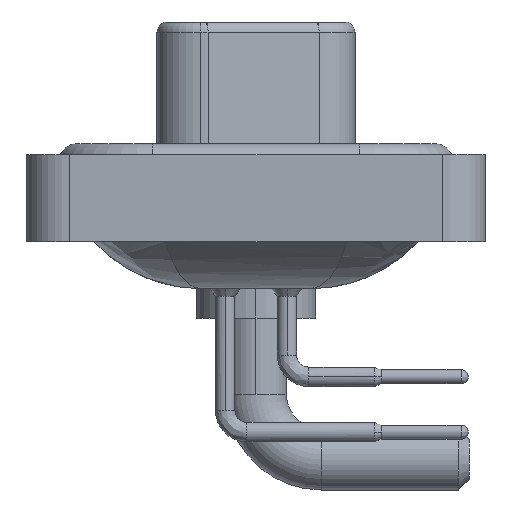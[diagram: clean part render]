
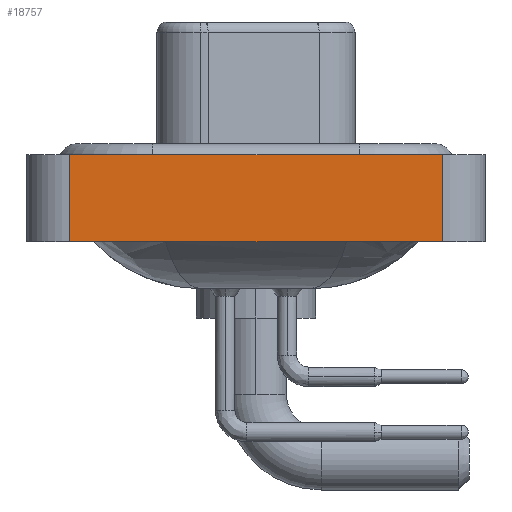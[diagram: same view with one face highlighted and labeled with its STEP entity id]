
A CAD part, left-side view. The second image highlights one B-rep face of the part: STEP entity #18757.
In plain terms, the highlighted planar face has unit normal (-1, 0, 0).
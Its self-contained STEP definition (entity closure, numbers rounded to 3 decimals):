
#782 = CARTESIAN_POINT ( 'NONE',  ( -7.35, -8.55, -3.6 ) ) ;
#877 = CARTESIAN_POINT ( 'NONE',  ( -7.35, -8.55, -3.6 ) ) ;
#1159 = CARTESIAN_POINT ( 'NONE',  ( -7.35, 8.55, 0.4 ) ) ;
#2008 = DIRECTION ( 'NONE',  ( 0., 0., 1. ) ) ;
#2098 = ORIENTED_EDGE ( 'NONE', *, *, #25594, .F. ) ;
#3463 = VERTEX_POINT ( 'NONE', #29595 ) ;
#3980 = LINE ( 'NONE', #877, #20474 ) ;
#4393 = LINE ( 'NONE', #14149, #15661 ) ;
#4493 = CARTESIAN_POINT ( 'NONE',  ( -7.35, -8.55, -3.6 ) ) ;
#5490 = VERTEX_POINT ( 'NONE', #4493 ) ;
#5574 = DIRECTION ( 'NONE',  ( -1., 0., 0. ) ) ;
#5680 = ORIENTED_EDGE ( 'NONE', *, *, #21581, .T. ) ;
#6449 = VERTEX_POINT ( 'NONE', #9210 ) ;
#6730 = EDGE_CURVE ( 'NONE', #5490, #6449, #8735, .T. ) ;
#7424 = VERTEX_POINT ( 'NONE', #1159 ) ;
#8735 = LINE ( 'NONE', #26713, #27895 ) ;
#9210 = CARTESIAN_POINT ( 'NONE',  ( -7.35, -8.55, 0.4 ) ) ;
#9489 = DIRECTION ( 'NONE',  ( 0., 0., 1. ) ) ;
#11653 = EDGE_LOOP ( 'NONE', ( #24681, #23798, #2098, #5680 ) ) ;
#13937 = AXIS2_PLACEMENT_3D ( 'NONE', #782, #5574, #9489 ) ;
#14149 = CARTESIAN_POINT ( 'NONE',  ( -7.35, 8.55, -3.6 ) ) ;
#14296 = DIRECTION ( 'NONE',  ( 0., 0., 1. ) ) ;
#15481 = DIRECTION ( 'NONE',  ( 0., -1., 0. ) ) ;
#15661 = VECTOR ( 'NONE', #14296, 1000. ) ;
#17111 = VECTOR ( 'NONE', #15481, 1000. ) ;
#17845 = CARTESIAN_POINT ( 'NONE',  ( -7.35, -8.55, 0.4 ) ) ;
#18003 = LINE ( 'NONE', #17845, #17111 ) ;
#18757 = ADVANCED_FACE ( 'NONE', ( #19067 ), #25639, .T. ) ;
#18961 = EDGE_CURVE ( 'NONE', #7424, #6449, #18003, .T. ) ;
#19067 = FACE_OUTER_BOUND ( 'NONE', #11653, .T. ) ;
#19863 = DIRECTION ( 'NONE',  ( 0., -1., 0. ) ) ;
#20474 = VECTOR ( 'NONE', #19863, 1000. ) ;
#21581 = EDGE_CURVE ( 'NONE', #3463, #5490, #3980, .T. ) ;
#23798 = ORIENTED_EDGE ( 'NONE', *, *, #18961, .F. ) ;
#24681 = ORIENTED_EDGE ( 'NONE', *, *, #6730, .T. ) ;
#25594 = EDGE_CURVE ( 'NONE', #3463, #7424, #4393, .T. ) ;
#25639 = PLANE ( 'NONE',  #13937 ) ;
#26713 = CARTESIAN_POINT ( 'NONE',  ( -7.35, -8.55, -3.6 ) ) ;
#27895 = VECTOR ( 'NONE', #2008, 1000. ) ;
#29595 = CARTESIAN_POINT ( 'NONE',  ( -7.35, 8.55, -3.6 ) ) ;
